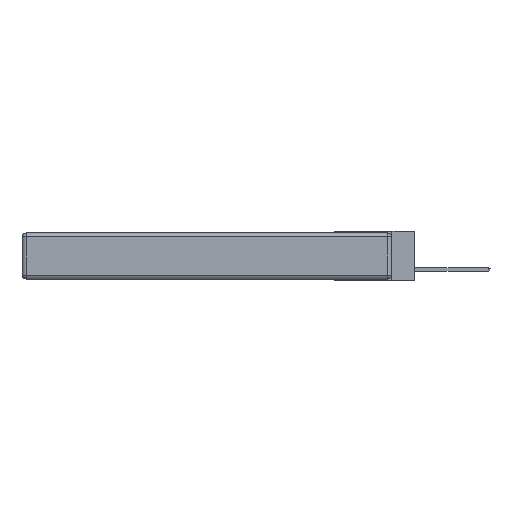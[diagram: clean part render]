
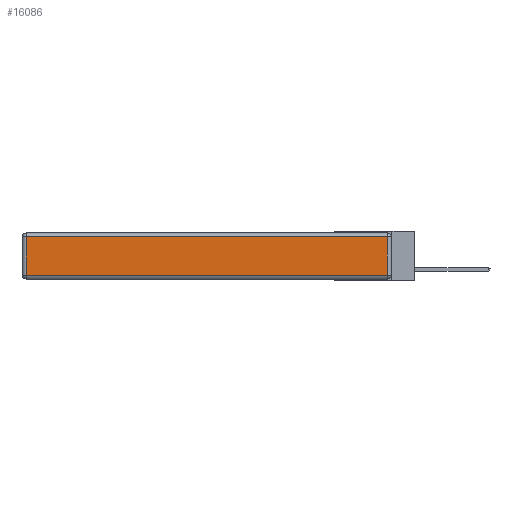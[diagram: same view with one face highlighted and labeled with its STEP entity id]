
A CAD part, left-side view. The second image highlights one B-rep face of the part: STEP entity #16086.
In plain terms, the highlighted planar face has unit normal (-1, 0, 0).
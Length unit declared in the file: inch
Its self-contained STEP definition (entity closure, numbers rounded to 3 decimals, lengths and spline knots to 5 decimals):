
#291 = VERTEX_POINT ( 'NONE', #30638 ) ;
#794 = VECTOR ( 'NONE', #17984, 39.37008 ) ;
#1882 = ORIENTED_EDGE ( 'NONE', *, *, #30317, .T. ) ;
#2183 = CARTESIAN_POINT ( 'NONE',  ( 0., 0.03, -0.03 ) ) ;
#2306 = ORIENTED_EDGE ( 'NONE', *, *, #23335, .T. ) ;
#2851 = DIRECTION ( 'NONE',  ( 0., -1., 0. ) ) ;
#3012 = LINE ( 'NONE', #15939, #21641 ) ;
#4038 = EDGE_CURVE ( 'NONE', #291, #8138, #16299, .T. ) ;
#5405 = EDGE_CURVE ( 'NONE', #21466, #291, #25095, .T. ) ;
#6660 = PLANE ( 'NONE',  #32360 ) ;
#6890 = CARTESIAN_POINT ( 'NONE',  ( 0., 0., -0.343 ) ) ;
#7932 = FACE_OUTER_BOUND ( 'NONE', #27662, .T. ) ;
#8138 = VERTEX_POINT ( 'NONE', #18166 ) ;
#8577 = ORIENTED_EDGE ( 'NONE', *, *, #5405, .T. ) ;
#10073 = ORIENTED_EDGE ( 'NONE', *, *, #4038, .T. ) ;
#12960 = CARTESIAN_POINT ( 'NONE',  ( 0., 2.72, -0.03 ) ) ;
#13031 = VECTOR ( 'NONE', #2851, 39.37008 ) ;
#13272 = CARTESIAN_POINT ( 'NONE',  ( 0., 0.03, -0.343 ) ) ;
#13286 = DIRECTION ( 'NONE',  ( 0., 1., 0. ) ) ;
#15061 = CARTESIAN_POINT ( 'NONE',  ( 0., 2.72, -0.343 ) ) ;
#15939 = CARTESIAN_POINT ( 'NONE',  ( 0., 2.75, -0.03 ) ) ;
#16086 = ADVANCED_FACE ( 'NONE', ( #7932 ), #6660, .T. ) ;
#16299 = LINE ( 'NONE', #28849, #13031 ) ;
#17984 = DIRECTION ( 'NONE',  ( 0., 0., -1. ) ) ;
#18166 = CARTESIAN_POINT ( 'NONE',  ( 0., 0.03, -0.313 ) ) ;
#21466 = VERTEX_POINT ( 'NONE', #12960 ) ;
#21557 = DIRECTION ( 'NONE',  ( 0., 0., 1. ) ) ;
#21641 = VECTOR ( 'NONE', #13286, 39.37008 ) ;
#22077 = VECTOR ( 'NONE', #21557, 39.37008 ) ;
#23335 = EDGE_CURVE ( 'NONE', #8138, #25994, #25704, .T. ) ;
#25095 = LINE ( 'NONE', #15061, #794 ) ;
#25704 = LINE ( 'NONE', #13272, #22077 ) ;
#25994 = VERTEX_POINT ( 'NONE', #2183 ) ;
#27662 = EDGE_LOOP ( 'NONE', ( #10073, #2306, #1882, #8577 ) ) ;
#28849 = CARTESIAN_POINT ( 'NONE',  ( 0., 0., -0.313 ) ) ;
#30190 = DIRECTION ( 'NONE',  ( -1., 0., 0. ) ) ;
#30317 = EDGE_CURVE ( 'NONE', #25994, #21466, #3012, .T. ) ;
#30638 = CARTESIAN_POINT ( 'NONE',  ( 0., 2.72, -0.313 ) ) ;
#32360 = AXIS2_PLACEMENT_3D ( 'NONE', #6890, #30190, #32550 ) ;
#32550 = DIRECTION ( 'NONE',  ( 0., 0., 1. ) ) ;
